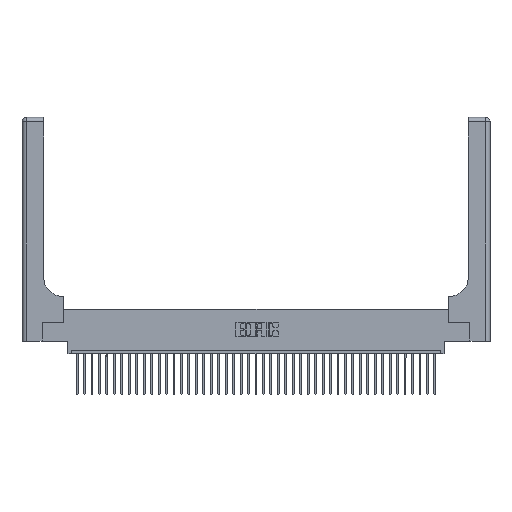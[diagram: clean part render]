
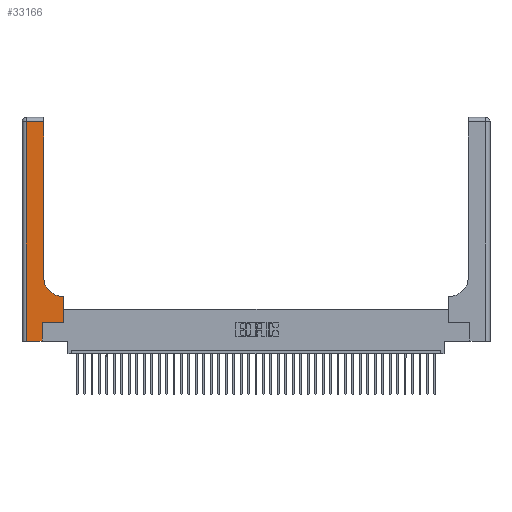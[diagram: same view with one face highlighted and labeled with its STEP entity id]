
A CAD part, top view. The second image highlights one B-rep face of the part: STEP entity #33166.
In plain terms, the highlighted planar face has unit normal (0, 0, 1).
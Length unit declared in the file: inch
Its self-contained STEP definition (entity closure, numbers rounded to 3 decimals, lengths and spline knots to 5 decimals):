
#1 = DIRECTION ( 'NONE',  ( 0., 0., -1. ) ) ;
#274 = EDGE_CURVE ( 'NONE', #13168, #30598, #10889, .T. ) ;
#557 = CARTESIAN_POINT ( 'NONE',  ( 0.5415, 0.6, 0.37 ) ) ;
#2295 = ORIENTED_EDGE ( 'NONE', *, *, #31537, .T. ) ;
#2738 = VERTEX_POINT ( 'NONE', #34437 ) ;
#2919 = EDGE_CURVE ( 'NONE', #23143, #7236, #34388, .T. ) ;
#3854 = DIRECTION ( 'NONE',  ( -1., 0., 0. ) ) ;
#4061 = DIRECTION ( 'NONE',  ( 0., 0., -1. ) ) ;
#4309 = EDGE_CURVE ( 'NONE', #7236, #40736, #33268, .T. ) ;
#4534 = DIRECTION ( 'NONE',  ( -1., 0., 0. ) ) ;
#6740 = PLANE ( 'NONE',  #7654 ) ;
#7236 = VERTEX_POINT ( 'NONE', #32768 ) ;
#7654 = AXIS2_PLACEMENT_3D ( 'NONE', #29367, #4061, #13494 ) ;
#8477 = DIRECTION ( 'NONE',  ( 0., 1., 0. ) ) ;
#8693 = DIRECTION ( 'NONE',  ( 0., 1., 0. ) ) ;
#8835 = VECTOR ( 'NONE', #18721, 39.37008 ) ;
#8969 = VERTEX_POINT ( 'NONE', #28960 ) ;
#9139 = CARTESIAN_POINT ( 'NONE',  ( 0.5585, 0.25, 0.37 ) ) ;
#9289 = CIRCLE ( 'NONE', #28115, 0.25 ) ;
#9450 = ORIENTED_EDGE ( 'NONE', *, *, #4309, .T. ) ;
#9828 = FACE_OUTER_BOUND ( 'NONE', #21189, .T. ) ;
#9915 = VECTOR ( 'NONE', #8693, 39.37008 ) ;
#10889 = LINE ( 'NONE', #33487, #17338 ) ;
#11766 = ORIENTED_EDGE ( 'NONE', *, *, #25612, .T. ) ;
#13168 = VERTEX_POINT ( 'NONE', #24775 ) ;
#13494 = DIRECTION ( 'NONE',  ( -1., 0., 0. ) ) ;
#13764 = VERTEX_POINT ( 'NONE', #557 ) ;
#14557 = VECTOR ( 'NONE', #19918, 39.37008 ) ;
#14601 = EDGE_CURVE ( 'NONE', #2738, #23143, #26870, .T. ) ;
#15421 = EDGE_CURVE ( 'NONE', #20915, #13168, #21320, .T. ) ;
#15422 = ORIENTED_EDGE ( 'NONE', *, *, #36275, .T. ) ;
#15944 = DIRECTION ( 'NONE',  ( 1., 0., 0. ) ) ;
#16315 = VECTOR ( 'NONE', #22586, 39.37008 ) ;
#17181 = ORIENTED_EDGE ( 'NONE', *, *, #2919, .T. ) ;
#17338 = VECTOR ( 'NONE', #17762, 39.37008 ) ;
#17762 = DIRECTION ( 'NONE',  ( 1., 0., 0. ) ) ;
#18108 = CARTESIAN_POINT ( 'NONE',  ( 0.06, 0., 0.37 ) ) ;
#18721 = DIRECTION ( 'NONE',  ( 0., 1., 0. ) ) ;
#19918 = DIRECTION ( 'NONE',  ( 1., 0., 0. ) ) ;
#20915 = VERTEX_POINT ( 'NONE', #30908 ) ;
#21189 = EDGE_LOOP ( 'NONE', ( #37334, #17181, #9450, #15422, #30008, #39420, #11766, #22717, #2295 ) ) ;
#21320 = LINE ( 'NONE', #27676, #36218 ) ;
#22451 = CARTESIAN_POINT ( 'NONE',  ( 0.06, 3., 0.37 ) ) ;
#22586 = DIRECTION ( 'NONE',  ( 0., -1., 0. ) ) ;
#22717 = ORIENTED_EDGE ( 'NONE', *, *, #24394, .T. ) ;
#23143 = VERTEX_POINT ( 'NONE', #32661 ) ;
#24394 = EDGE_CURVE ( 'NONE', #8969, #13764, #38531, .T. ) ;
#24775 = CARTESIAN_POINT ( 'NONE',  ( 0.269, 0.25, 0.37 ) ) ;
#25110 = VECTOR ( 'NONE', #3854, 39.37008 ) ;
#25568 = LINE ( 'NONE', #28450, #14557 ) ;
#25612 = EDGE_CURVE ( 'NONE', #30598, #8969, #38217, .T. ) ;
#26870 = LINE ( 'NONE', #39295, #9915 ) ;
#27676 = CARTESIAN_POINT ( 'NONE',  ( 0.269, 0., 0.37 ) ) ;
#28115 = AXIS2_PLACEMENT_3D ( 'NONE', #38006, #1, #15944 ) ;
#28450 = CARTESIAN_POINT ( 'NONE',  ( 0., 0., 0.37 ) ) ;
#28960 = CARTESIAN_POINT ( 'NONE',  ( 0.5585, 0.6, 0.37 ) ) ;
#29367 = CARTESIAN_POINT ( 'NONE',  ( 0., 3., 0.37 ) ) ;
#30008 = ORIENTED_EDGE ( 'NONE', *, *, #15421, .T. ) ;
#30598 = VERTEX_POINT ( 'NONE', #33350 ) ;
#30908 = CARTESIAN_POINT ( 'NONE',  ( 0.269, 0., 0.37 ) ) ;
#31537 = EDGE_CURVE ( 'NONE', #13764, #2738, #9289, .T. ) ;
#32661 = CARTESIAN_POINT ( 'NONE',  ( 0.2915, 2.94, 0.37 ) ) ;
#32768 = CARTESIAN_POINT ( 'NONE',  ( 0.06, 2.94, 0.37 ) ) ;
#33166 = ADVANCED_FACE ( 'NONE', ( #9828 ), #6740, .F. ) ;
#33268 = LINE ( 'NONE', #22451, #16315 ) ;
#33350 = CARTESIAN_POINT ( 'NONE',  ( 0.5585, 0.25, 0.37 ) ) ;
#33487 = CARTESIAN_POINT ( 'NONE',  ( 0.269, 0.25, 0.37 ) ) ;
#34388 = LINE ( 'NONE', #39476, #35359 ) ;
#34437 = CARTESIAN_POINT ( 'NONE',  ( 0.2915, 0.85, 0.37 ) ) ;
#35359 = VECTOR ( 'NONE', #4534, 39.37008 ) ;
#36218 = VECTOR ( 'NONE', #8477, 39.37008 ) ;
#36275 = EDGE_CURVE ( 'NONE', #40736, #20915, #25568, .T. ) ;
#37334 = ORIENTED_EDGE ( 'NONE', *, *, #14601, .T. ) ;
#38006 = CARTESIAN_POINT ( 'NONE',  ( 0.5415, 0.85, 0.37 ) ) ;
#38217 = LINE ( 'NONE', #9139, #8835 ) ;
#38516 = CARTESIAN_POINT ( 'NONE',  ( 0.2915, 0.6, 0.37 ) ) ;
#38531 = LINE ( 'NONE', #38516, #25110 ) ;
#39295 = CARTESIAN_POINT ( 'NONE',  ( 0.2915, 3., 0.37 ) ) ;
#39420 = ORIENTED_EDGE ( 'NONE', *, *, #274, .T. ) ;
#39476 = CARTESIAN_POINT ( 'NONE',  ( 0., 2.94, 0.37 ) ) ;
#40736 = VERTEX_POINT ( 'NONE', #18108 ) ;
